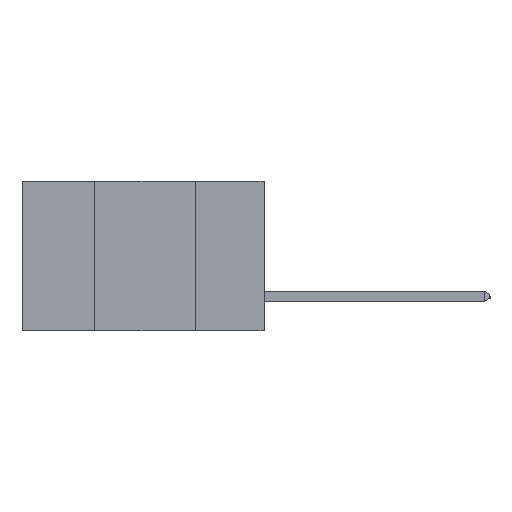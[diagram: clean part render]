
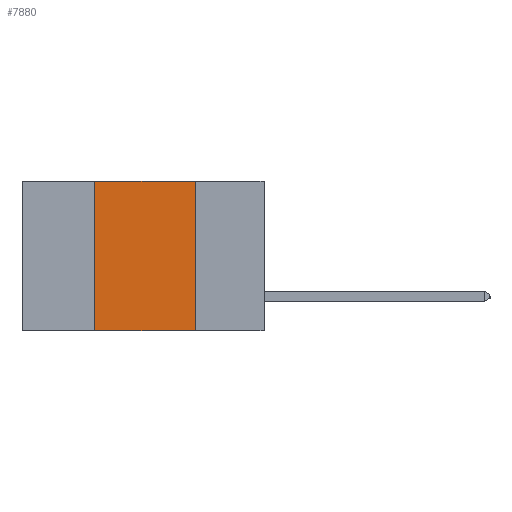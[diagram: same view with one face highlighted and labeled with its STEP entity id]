
A CAD part, left-side view. The second image highlights one B-rep face of the part: STEP entity #7880.
In plain terms, the highlighted planar face has unit normal (-1, 0, 0).
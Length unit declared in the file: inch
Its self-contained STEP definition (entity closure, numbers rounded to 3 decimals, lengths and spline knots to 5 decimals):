
#618 = CARTESIAN_POINT ( 'NONE',  ( 0., 0.42, 0. ) ) ;
#767 = VERTEX_POINT ( 'NONE', #7342 ) ;
#858 = ORIENTED_EDGE ( 'NONE', *, *, #10467, .F. ) ;
#1144 = EDGE_LOOP ( 'NONE', ( #858, #2236, #4930, #6079 ) ) ;
#1241 = VECTOR ( 'NONE', #10528, 39.37008 ) ;
#1897 = FACE_OUTER_BOUND ( 'NONE', #1144, .T. ) ;
#2236 = ORIENTED_EDGE ( 'NONE', *, *, #10606, .F. ) ;
#2394 = CARTESIAN_POINT ( 'NONE',  ( 0., 0.17, 0. ) ) ;
#2873 = VECTOR ( 'NONE', #5603, 39.37008 ) ;
#3023 = CARTESIAN_POINT ( 'NONE',  ( 0., 0.42, -0.37 ) ) ;
#3334 = AXIS2_PLACEMENT_3D ( 'NONE', #9012, #10722, #5451 ) ;
#3929 = CARTESIAN_POINT ( 'NONE',  ( 0., 0.17, -0.37 ) ) ;
#4028 = LINE ( 'NONE', #2394, #1241 ) ;
#4491 = PLANE ( 'NONE',  #3334 ) ;
#4930 = ORIENTED_EDGE ( 'NONE', *, *, #9325, .F. ) ;
#5127 = EDGE_CURVE ( 'NONE', #8379, #11368, #10070, .T. ) ;
#5451 = DIRECTION ( 'NONE',  ( 0., 0., -1. ) ) ;
#5603 = DIRECTION ( 'NONE',  ( 0., -1., 0. ) ) ;
#5623 = CARTESIAN_POINT ( 'NONE',  ( 0., 0.6, -0.37 ) ) ;
#6079 = ORIENTED_EDGE ( 'NONE', *, *, #5127, .T. ) ;
#6242 = DIRECTION ( 'NONE',  ( 0., 0., 1. ) ) ;
#6375 = DIRECTION ( 'NONE',  ( 0., -1., 0. ) ) ;
#7215 = VECTOR ( 'NONE', #6375, 39.37008 ) ;
#7342 = CARTESIAN_POINT ( 'NONE',  ( 0., 0.42, 0. ) ) ;
#7880 = ADVANCED_FACE ( 'NONE', ( #1897 ), #4491, .F. ) ;
#8379 = VERTEX_POINT ( 'NONE', #3023 ) ;
#9012 = CARTESIAN_POINT ( 'NONE',  ( 0., 0.6, 0. ) ) ;
#9267 = LINE ( 'NONE', #11543, #7215 ) ;
#9299 = VECTOR ( 'NONE', #6242, 39.37008 ) ;
#9325 = EDGE_CURVE ( 'NONE', #8379, #767, #11538, .T. ) ;
#9819 = CARTESIAN_POINT ( 'NONE',  ( 0., 0.17, 0. ) ) ;
#10070 = LINE ( 'NONE', #5623, #2873 ) ;
#10467 = EDGE_CURVE ( 'NONE', #10580, #11368, #4028, .T. ) ;
#10528 = DIRECTION ( 'NONE',  ( 0., 0., -1. ) ) ;
#10580 = VERTEX_POINT ( 'NONE', #9819 ) ;
#10606 = EDGE_CURVE ( 'NONE', #767, #10580, #9267, .T. ) ;
#10722 = DIRECTION ( 'NONE',  ( 1., 0., 0. ) ) ;
#11368 = VERTEX_POINT ( 'NONE', #3929 ) ;
#11538 = LINE ( 'NONE', #618, #9299 ) ;
#11543 = CARTESIAN_POINT ( 'NONE',  ( 0., 0.6, 0. ) ) ;
